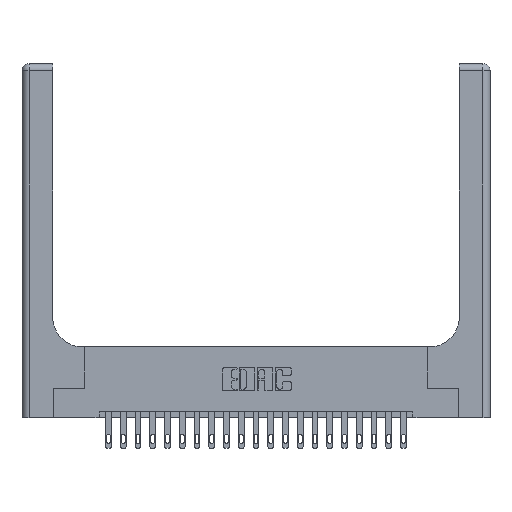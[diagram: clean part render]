
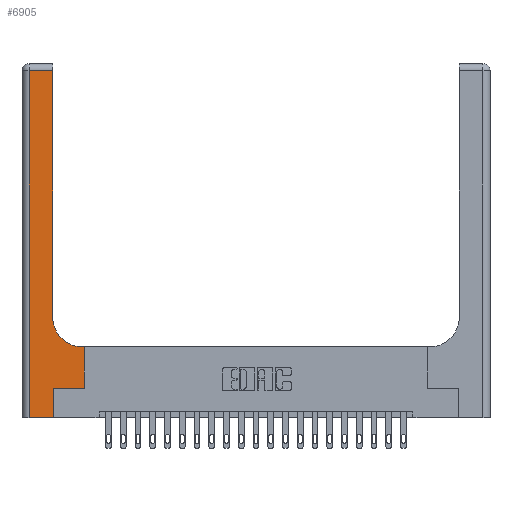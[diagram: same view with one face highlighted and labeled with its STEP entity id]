
A CAD part, top view. The second image highlights one B-rep face of the part: STEP entity #6905.
In plain terms, the highlighted planar face has unit normal (0, 0, 1).
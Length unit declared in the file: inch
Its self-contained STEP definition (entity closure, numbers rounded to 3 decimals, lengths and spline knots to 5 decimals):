
#164 = ORIENTED_EDGE ( 'NONE', *, *, #18312, .T. ) ;
#300 = DIRECTION ( 'NONE',  ( 0., 1., 0. ) ) ;
#786 = VECTOR ( 'NONE', #300, 39.37008 ) ;
#904 = LINE ( 'NONE', #16460, #8400 ) ;
#1014 = DIRECTION ( 'NONE',  ( -1., 0., 0. ) ) ;
#1946 = CIRCLE ( 'NONE', #20866, 0.25 ) ;
#2591 = DIRECTION ( 'NONE',  ( 1., 0., 0. ) ) ;
#3093 = LINE ( 'NONE', #9900, #21311 ) ;
#3757 = CARTESIAN_POINT ( 'NONE',  ( 0.528, 0.6, 0.37 ) ) ;
#3952 = LINE ( 'NONE', #17816, #19483 ) ;
#4111 = CARTESIAN_POINT ( 'NONE',  ( 0.06, 0., 0.37 ) ) ;
#4271 = EDGE_CURVE ( 'NONE', #14961, #15846, #10480, .T. ) ;
#4759 = DIRECTION ( 'NONE',  ( 0., 0., -1. ) ) ;
#5014 = EDGE_CURVE ( 'NONE', #15846, #8578, #13437, .T. ) ;
#5236 = VERTEX_POINT ( 'NONE', #19576 ) ;
#5626 = EDGE_CURVE ( 'NONE', #9195, #21193, #21840, .T. ) ;
#6112 = DIRECTION ( 'NONE',  ( -1., 0., 0. ) ) ;
#6905 = ADVANCED_FACE ( 'NONE', ( #13254 ), #16612, .F. ) ;
#7455 = CARTESIAN_POINT ( 'NONE',  ( 0.51, 0.85, 0.37 ) ) ;
#7558 = ORIENTED_EDGE ( 'NONE', *, *, #9279, .T. ) ;
#8400 = VECTOR ( 'NONE', #1014, 39.37008 ) ;
#8578 = VERTEX_POINT ( 'NONE', #10195 ) ;
#8789 = CARTESIAN_POINT ( 'NONE',  ( 0.528, 0.25, 0.37 ) ) ;
#8805 = ORIENTED_EDGE ( 'NONE', *, *, #19267, .T. ) ;
#8852 = EDGE_CURVE ( 'NONE', #8578, #14962, #21576, .T. ) ;
#9140 = AXIS2_PLACEMENT_3D ( 'NONE', #20073, #4759, #6112 ) ;
#9195 = VERTEX_POINT ( 'NONE', #8789 ) ;
#9279 = EDGE_CURVE ( 'NONE', #14962, #14460, #3952, .T. ) ;
#9484 = CARTESIAN_POINT ( 'NONE',  ( 0.26, 2.94, 0.37 ) ) ;
#9900 = CARTESIAN_POINT ( 'NONE',  ( 0.265, 0.25, 0.37 ) ) ;
#9961 = DIRECTION ( 'NONE',  ( -1., 0., 0. ) ) ;
#10146 = DIRECTION ( 'NONE',  ( 0., 1., 0. ) ) ;
#10195 = CARTESIAN_POINT ( 'NONE',  ( 0.06, 2.94, 0.37 ) ) ;
#10480 = LINE ( 'NONE', #17206, #786 ) ;
#10914 = VECTOR ( 'NONE', #9961, 39.37008 ) ;
#11205 = ORIENTED_EDGE ( 'NONE', *, *, #4271, .T. ) ;
#11787 = DIRECTION ( 'NONE',  ( 0., 1., 0. ) ) ;
#12663 = VECTOR ( 'NONE', #13091, 39.37008 ) ;
#13091 = DIRECTION ( 'NONE',  ( 0., -1., 0. ) ) ;
#13158 = CARTESIAN_POINT ( 'NONE',  ( 0.51, 0.6, 0.37 ) ) ;
#13254 = FACE_OUTER_BOUND ( 'NONE', #18565, .T. ) ;
#13256 = ORIENTED_EDGE ( 'NONE', *, *, #5014, .T. ) ;
#13437 = LINE ( 'NONE', #13543, #10914 ) ;
#13512 = ORIENTED_EDGE ( 'NONE', *, *, #8852, .T. ) ;
#13543 = CARTESIAN_POINT ( 'NONE',  ( 0., 2.94, 0.37 ) ) ;
#13651 = VECTOR ( 'NONE', #10146, 39.37008 ) ;
#14460 = VERTEX_POINT ( 'NONE', #20776 ) ;
#14830 = EDGE_CURVE ( 'NONE', #14460, #5236, #17196, .T. ) ;
#14961 = VERTEX_POINT ( 'NONE', #17529 ) ;
#14962 = VERTEX_POINT ( 'NONE', #4111 ) ;
#15573 = VECTOR ( 'NONE', #11787, 39.37008 ) ;
#15846 = VERTEX_POINT ( 'NONE', #9484 ) ;
#15967 = ORIENTED_EDGE ( 'NONE', *, *, #5626, .T. ) ;
#16027 = CARTESIAN_POINT ( 'NONE',  ( 0.265, 0., 0.37 ) ) ;
#16057 = DIRECTION ( 'NONE',  ( 1., 0., 0. ) ) ;
#16460 = CARTESIAN_POINT ( 'NONE',  ( 0.26, 0.6, 0.37 ) ) ;
#16612 = PLANE ( 'NONE',  #9140 ) ;
#16738 = DIRECTION ( 'NONE',  ( 1., 0., 0. ) ) ;
#16977 = ORIENTED_EDGE ( 'NONE', *, *, #17780, .T. ) ;
#17196 = LINE ( 'NONE', #16027, #13651 ) ;
#17206 = CARTESIAN_POINT ( 'NONE',  ( 0.26, 3., 0.37 ) ) ;
#17529 = CARTESIAN_POINT ( 'NONE',  ( 0.26, 0.85, 0.37 ) ) ;
#17780 = EDGE_CURVE ( 'NONE', #19161, #14961, #1946, .T. ) ;
#17816 = CARTESIAN_POINT ( 'NONE',  ( 0., 0., 0.37 ) ) ;
#18312 = EDGE_CURVE ( 'NONE', #21193, #19161, #904, .T. ) ;
#18565 = EDGE_LOOP ( 'NONE', ( #11205, #13256, #13512, #7558, #21630, #8805, #15967, #164, #16977 ) ) ;
#19161 = VERTEX_POINT ( 'NONE', #13158 ) ;
#19267 = EDGE_CURVE ( 'NONE', #5236, #9195, #3093, .T. ) ;
#19483 = VECTOR ( 'NONE', #2591, 39.37008 ) ;
#19512 = DIRECTION ( 'NONE',  ( 0., 0., -1. ) ) ;
#19576 = CARTESIAN_POINT ( 'NONE',  ( 0.265, 0.25, 0.37 ) ) ;
#20022 = CARTESIAN_POINT ( 'NONE',  ( 0.06, 3., 0.37 ) ) ;
#20073 = CARTESIAN_POINT ( 'NONE',  ( 0., 3., 0.37 ) ) ;
#20285 = CARTESIAN_POINT ( 'NONE',  ( 0.528, 0.25, 0.37 ) ) ;
#20776 = CARTESIAN_POINT ( 'NONE',  ( 0.265, 0., 0.37 ) ) ;
#20866 = AXIS2_PLACEMENT_3D ( 'NONE', #7455, #19512, #16057 ) ;
#21193 = VERTEX_POINT ( 'NONE', #3757 ) ;
#21311 = VECTOR ( 'NONE', #16738, 39.37008 ) ;
#21576 = LINE ( 'NONE', #20022, #12663 ) ;
#21630 = ORIENTED_EDGE ( 'NONE', *, *, #14830, .T. ) ;
#21840 = LINE ( 'NONE', #20285, #15573 ) ;
